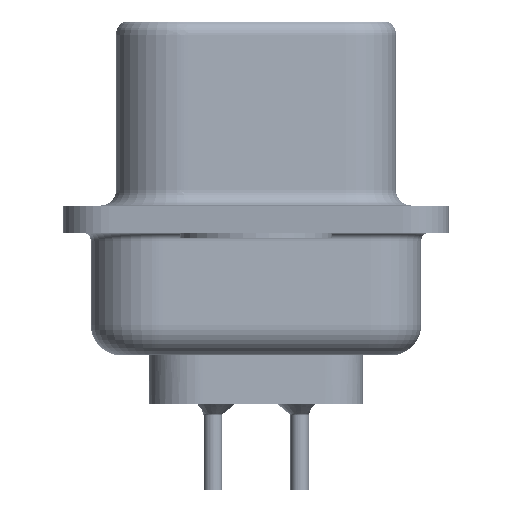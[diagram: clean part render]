
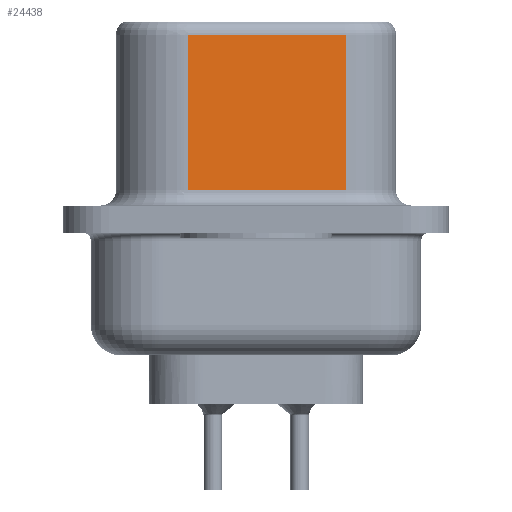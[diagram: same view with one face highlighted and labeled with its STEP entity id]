
A CAD part, left-side view. The second image highlights one B-rep face of the part: STEP entity #24438.
In plain terms, the highlighted planar face has unit normal (-0.985, -0.174, 0).
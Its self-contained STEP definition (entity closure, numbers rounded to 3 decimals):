
#1167 = VERTEX_POINT ( 'NONE', #21667 ) ;
#2032 = CARTESIAN_POINT ( 'NONE',  ( 3.67, 2.233, 6.52 ) ) ;
#2588 = CARTESIAN_POINT ( 'NONE',  ( 4.58, -2.927, 6.52 ) ) ;
#2906 = ORIENTED_EDGE ( 'NONE', *, *, #4959, .T. ) ;
#3451 = EDGE_CURVE ( 'NONE', #1167, #17729, #7623, .T. ) ;
#4959 = EDGE_CURVE ( 'NONE', #17729, #6087, #26958, .T. ) ;
#5803 = AXIS2_PLACEMENT_3D ( 'NONE', #2588, #9031, #23935 ) ;
#6087 = VERTEX_POINT ( 'NONE', #26149 ) ;
#6845 = EDGE_CURVE ( 'NONE', #6087, #24665, #27519, .T. ) ;
#7623 = LINE ( 'NONE', #24197, #8982 ) ;
#8982 = VECTOR ( 'NONE', #23831, 1000. ) ;
#9031 = DIRECTION ( 'NONE',  ( 0.985, 0.174, 0. ) ) ;
#9110 = ORIENTED_EDGE ( 'NONE', *, *, #18632, .F. ) ;
#10657 = LINE ( 'NONE', #21371, #26988 ) ;
#11549 = ORIENTED_EDGE ( 'NONE', *, *, #6845, .T. ) ;
#11990 = CARTESIAN_POINT ( 'NONE',  ( 4.58, -2.927, 0.95 ) ) ;
#12130 = CARTESIAN_POINT ( 'NONE',  ( 4.58, -2.927, 0.95 ) ) ;
#12568 = DIRECTION ( 'NONE',  ( 0., 0., -1. ) ) ;
#17442 = CARTESIAN_POINT ( 'NONE',  ( 3.67, 2.233, 6.02 ) ) ;
#17592 = FACE_OUTER_BOUND ( 'NONE', #18097, .T. ) ;
#17729 = VERTEX_POINT ( 'NONE', #17442 ) ;
#18097 = EDGE_LOOP ( 'NONE', ( #9110, #21240, #2906, #11549 ) ) ;
#18632 = EDGE_CURVE ( 'NONE', #1167, #24665, #10657, .T. ) ;
#21240 = ORIENTED_EDGE ( 'NONE', *, *, #3451, .T. ) ;
#21371 = CARTESIAN_POINT ( 'NONE',  ( 4.58, -2.927, 6.52 ) ) ;
#21667 = CARTESIAN_POINT ( 'NONE',  ( 4.58, -2.927, 6.02 ) ) ;
#21849 = VECTOR ( 'NONE', #27061, 1000. ) ;
#23482 = DIRECTION ( 'NONE',  ( 0., 0., -1. ) ) ;
#23831 = DIRECTION ( 'NONE',  ( -0.174, 0.985, 0. ) ) ;
#23839 = PLANE ( 'NONE',  #5803 ) ;
#23935 = DIRECTION ( 'NONE',  ( -0.174, 0.985, 0. ) ) ;
#24197 = CARTESIAN_POINT ( 'NONE',  ( 4.58, -2.927, 6.02 ) ) ;
#24438 = ADVANCED_FACE ( 'NONE', ( #17592 ), #23839, .F. ) ;
#24665 = VERTEX_POINT ( 'NONE', #11990 ) ;
#26149 = CARTESIAN_POINT ( 'NONE',  ( 3.67, 2.233, 0.95 ) ) ;
#26280 = VECTOR ( 'NONE', #12568, 1000. ) ;
#26958 = LINE ( 'NONE', #2032, #26280 ) ;
#26988 = VECTOR ( 'NONE', #23482, 1000. ) ;
#27061 = DIRECTION ( 'NONE',  ( 0.174, -0.985, 0. ) ) ;
#27519 = LINE ( 'NONE', #12130, #21849 ) ;
